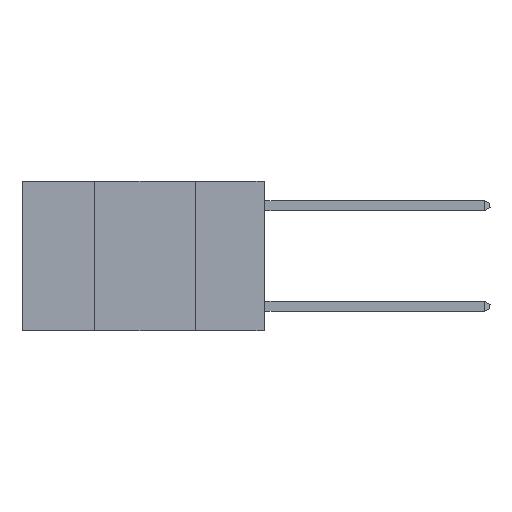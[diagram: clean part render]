
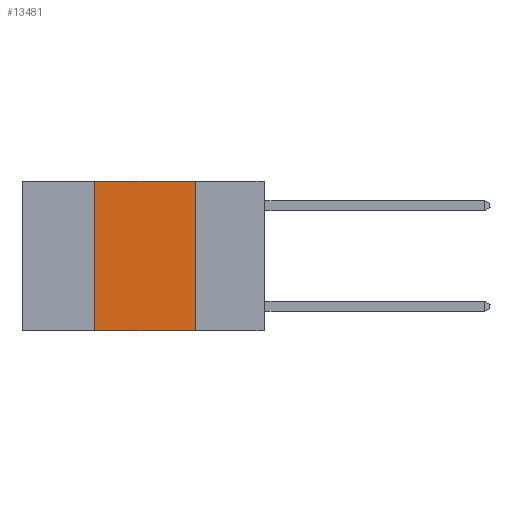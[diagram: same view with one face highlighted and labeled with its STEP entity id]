
A CAD part, left-side view. The second image highlights one B-rep face of the part: STEP entity #13481.
In plain terms, the highlighted planar face has unit normal (-1, 0, 0).
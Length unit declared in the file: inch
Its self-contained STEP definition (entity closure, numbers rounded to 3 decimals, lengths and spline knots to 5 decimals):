
#405 = PLANE ( 'NONE',  #5519 ) ;
#636 = CARTESIAN_POINT ( 'NONE',  ( 0., 0.6, 0. ) ) ;
#1058 = DIRECTION ( 'NONE',  ( 0., 0., -1. ) ) ;
#1205 = CARTESIAN_POINT ( 'NONE',  ( 0., 0.42, 0. ) ) ;
#1360 = EDGE_CURVE ( 'NONE', #11195, #1414, #2179, .T. ) ;
#1414 = VERTEX_POINT ( 'NONE', #9154 ) ;
#2179 = LINE ( 'NONE', #636, #6716 ) ;
#2800 = DIRECTION ( 'NONE',  ( 0., -1., 0. ) ) ;
#3869 = ORIENTED_EDGE ( 'NONE', *, *, #12910, .T. ) ;
#4231 = FACE_OUTER_BOUND ( 'NONE', #11795, .T. ) ;
#4316 = DIRECTION ( 'NONE',  ( 0., 0., -1. ) ) ;
#4503 = DIRECTION ( 'NONE',  ( 1., 0., 0. ) ) ;
#4730 = DIRECTION ( 'NONE',  ( 0., -1., 0. ) ) ;
#5200 = VECTOR ( 'NONE', #11296, 39.37008 ) ;
#5519 = AXIS2_PLACEMENT_3D ( 'NONE', #16890, #4503, #4316 ) ;
#5799 = VERTEX_POINT ( 'NONE', #15290 ) ;
#5812 = CARTESIAN_POINT ( 'NONE',  ( 0., 0.42, 0. ) ) ;
#6080 = LINE ( 'NONE', #5812, #5200 ) ;
#6384 = VERTEX_POINT ( 'NONE', #9857 ) ;
#6661 = EDGE_CURVE ( 'NONE', #1414, #5799, #17621, .T. ) ;
#6716 = VECTOR ( 'NONE', #4730, 39.37008 ) ;
#6812 = LINE ( 'NONE', #17643, #17063 ) ;
#7948 = CARTESIAN_POINT ( 'NONE',  ( 0., 0.17, 0. ) ) ;
#8945 = ORIENTED_EDGE ( 'NONE', *, *, #10012, .F. ) ;
#9154 = CARTESIAN_POINT ( 'NONE',  ( 0., 0.17, 0. ) ) ;
#9857 = CARTESIAN_POINT ( 'NONE',  ( 0., 0.42, -0.37 ) ) ;
#10012 = EDGE_CURVE ( 'NONE', #6384, #11195, #6080, .T. ) ;
#10403 = VECTOR ( 'NONE', #1058, 39.37008 ) ;
#11195 = VERTEX_POINT ( 'NONE', #1205 ) ;
#11296 = DIRECTION ( 'NONE',  ( 0., 0., 1. ) ) ;
#11795 = EDGE_LOOP ( 'NONE', ( #17058, #13498, #8945, #3869 ) ) ;
#12910 = EDGE_CURVE ( 'NONE', #6384, #5799, #6812, .T. ) ;
#13481 = ADVANCED_FACE ( 'NONE', ( #4231 ), #405, .F. ) ;
#13498 = ORIENTED_EDGE ( 'NONE', *, *, #1360, .F. ) ;
#15290 = CARTESIAN_POINT ( 'NONE',  ( 0., 0.17, -0.37 ) ) ;
#16890 = CARTESIAN_POINT ( 'NONE',  ( 0., 0.6, 0. ) ) ;
#17058 = ORIENTED_EDGE ( 'NONE', *, *, #6661, .F. ) ;
#17063 = VECTOR ( 'NONE', #2800, 39.37008 ) ;
#17621 = LINE ( 'NONE', #7948, #10403 ) ;
#17643 = CARTESIAN_POINT ( 'NONE',  ( 0., 0.6, -0.37 ) ) ;
